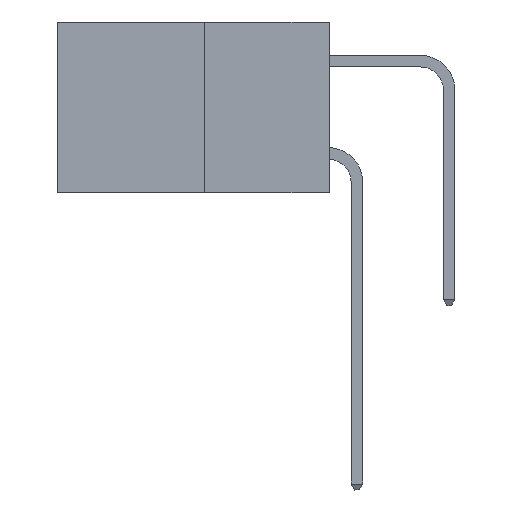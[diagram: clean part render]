
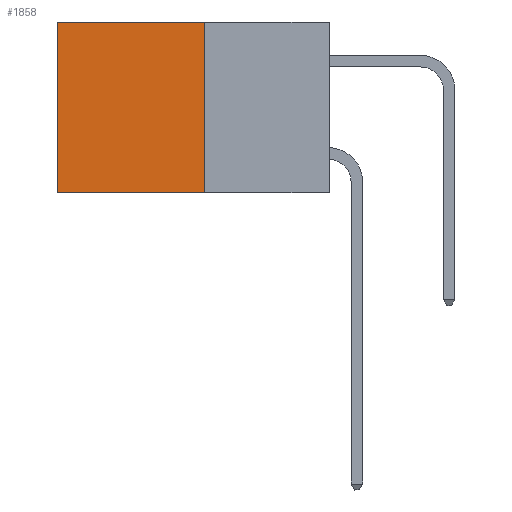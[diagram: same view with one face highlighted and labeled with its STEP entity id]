
A CAD part, left-side view. The second image highlights one B-rep face of the part: STEP entity #1858.
In plain terms, the highlighted planar face has unit normal (-1, 0, 0).
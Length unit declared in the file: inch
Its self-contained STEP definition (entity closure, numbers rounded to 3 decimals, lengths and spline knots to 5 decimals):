
#611 = LINE ( 'NONE', #1433, #11427 ) ;
#1194 = EDGE_CURVE ( 'NONE', #17170, #15572, #611, .T. ) ;
#1433 = CARTESIAN_POINT ( 'NONE',  ( 0.277, 0.27, -0.37 ) ) ;
#1554 = VERTEX_POINT ( 'NONE', #8659 ) ;
#1571 = ORIENTED_EDGE ( 'NONE', *, *, #8435, .F. ) ;
#1740 = CARTESIAN_POINT ( 'NONE',  ( 0.277, 0.59, 0. ) ) ;
#1858 = ADVANCED_FACE ( 'NONE', ( #14979 ), #2047, .F. ) ;
#1872 = AXIS2_PLACEMENT_3D ( 'NONE', #4971, #15294, #6437 ) ;
#2047 = PLANE ( 'NONE',  #1872 ) ;
#3864 = CARTESIAN_POINT ( 'NONE',  ( 0.277, 0.27, -0.37 ) ) ;
#4971 = CARTESIAN_POINT ( 'NONE',  ( 0.277, 0.27, -0.37 ) ) ;
#5044 = EDGE_CURVE ( 'NONE', #1554, #18183, #15974, .T. ) ;
#5754 = ORIENTED_EDGE ( 'NONE', *, *, #10500, .T. ) ;
#6134 = CARTESIAN_POINT ( 'NONE',  ( 0.277, 0.59, -0.37 ) ) ;
#6437 = DIRECTION ( 'NONE',  ( 0., 0., -1. ) ) ;
#7896 = CARTESIAN_POINT ( 'NONE',  ( 0.277, 0.59, -0.37 ) ) ;
#8435 = EDGE_CURVE ( 'NONE', #1554, #17170, #11516, .T. ) ;
#8659 = CARTESIAN_POINT ( 'NONE',  ( 0.277, 0.27, 0. ) ) ;
#9176 = DIRECTION ( 'NONE',  ( 0., 1., 0. ) ) ;
#10262 = VECTOR ( 'NONE', #16737, 39.37008 ) ;
#10500 = EDGE_CURVE ( 'NONE', #18183, #15572, #14188, .T. ) ;
#11057 = VECTOR ( 'NONE', #18357, 39.37008 ) ;
#11427 = VECTOR ( 'NONE', #11667, 39.37008 ) ;
#11516 = LINE ( 'NONE', #16853, #11057 ) ;
#11622 = VECTOR ( 'NONE', #9176, 39.37008 ) ;
#11667 = DIRECTION ( 'NONE',  ( 0., 1., 0. ) ) ;
#11690 = EDGE_LOOP ( 'NONE', ( #5754, #12810, #1571, #16218 ) ) ;
#12810 = ORIENTED_EDGE ( 'NONE', *, *, #1194, .F. ) ;
#14188 = LINE ( 'NONE', #7896, #10262 ) ;
#14979 = FACE_OUTER_BOUND ( 'NONE', #11690, .T. ) ;
#15091 = CARTESIAN_POINT ( 'NONE',  ( 0.277, 0.27, 0. ) ) ;
#15294 = DIRECTION ( 'NONE',  ( 1., 0., 0. ) ) ;
#15572 = VERTEX_POINT ( 'NONE', #6134 ) ;
#15974 = LINE ( 'NONE', #15091, #11622 ) ;
#16218 = ORIENTED_EDGE ( 'NONE', *, *, #5044, .T. ) ;
#16737 = DIRECTION ( 'NONE',  ( 0., 0., -1. ) ) ;
#16853 = CARTESIAN_POINT ( 'NONE',  ( 0.277, 0.27, -0.37 ) ) ;
#17170 = VERTEX_POINT ( 'NONE', #3864 ) ;
#18183 = VERTEX_POINT ( 'NONE', #1740 ) ;
#18357 = DIRECTION ( 'NONE',  ( 0., 0., -1. ) ) ;
